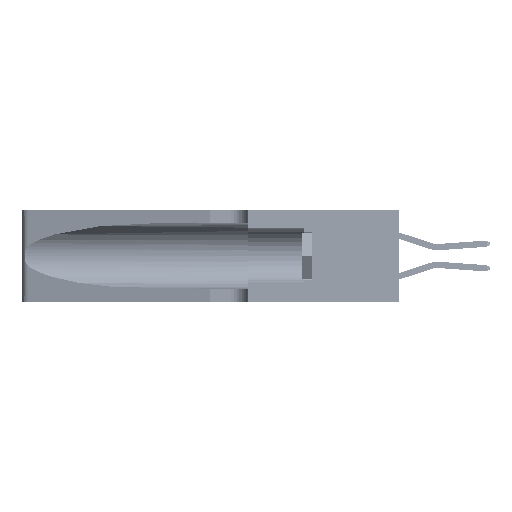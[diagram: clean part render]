
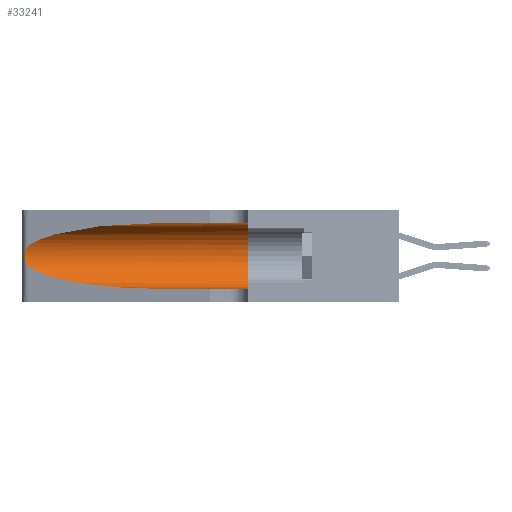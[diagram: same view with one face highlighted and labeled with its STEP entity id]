
A CAD part, left-side view. The second image highlights one B-rep face of the part: STEP entity #33241.
In plain terms, the highlighted cylindrical face has radius 3.308 mm (diameter 6.617 mm), a partial arc.
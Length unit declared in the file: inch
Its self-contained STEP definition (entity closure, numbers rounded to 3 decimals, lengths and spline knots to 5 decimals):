
#646 = CARTESIAN_POINT ( 'NONE',  ( 0.25555, 1.22994, 0.2215 ) ) ;
#1185 = DIRECTION ( 'NONE',  ( 0., -1., 0. ) ) ;
#1906 = VERTEX_POINT ( 'NONE', #7540 ) ;
#3377 = CIRCLE ( 'NONE', #4117, 0.13025 ) ;
#4117 = AXIS2_PLACEMENT_3D ( 'NONE', #32071, #7719, #36002 ) ;
#4422 = CARTESIAN_POINT ( 'NONE',  ( 0.25854, 1.2359, 0.20912 ) ) ;
#5748 = DIRECTION ( 'NONE',  ( 0., -1., 0. ) ) ;
#6317 = ORIENTED_EDGE ( 'NONE', *, *, #47443, .F. ) ;
#7099 = EDGE_CURVE ( 'NONE', #12326, #1906, #45762, .T. ) ;
#7443 = CARTESIAN_POINT ( 'NONE',  ( 0.18966, 0.96281, 0.05475 ) ) ;
#7540 = CARTESIAN_POINT ( 'NONE',  ( 0.1305, 0.35, 0.05475 ) ) ;
#7633 = CARTESIAN_POINT ( 'NONE',  ( 0.1305, 0.72297, 0.05475 ) ) ;
#7719 = DIRECTION ( 'NONE',  ( 0., 1., 0. ) ) ;
#8078 = CARTESIAN_POINT ( 'NONE',  ( 0.25487, 1.22718, 0.14631 ) ) ;
#8107 = EDGE_CURVE ( 'NONE', #32975, #12326, #27129, .T. ) ;
#8159 = ORIENTED_EDGE ( 'NONE', *, *, #41461, .F. ) ;
#8534 = CARTESIAN_POINT ( 'NONE',  ( 0.26075, 1.23896, 0.19203 ) ) ;
#9354 = AXIS2_PLACEMENT_3D ( 'NONE', #25885, #5748, #42400 ) ;
#9576 = FACE_OUTER_BOUND ( 'NONE', #43504, .T. ) ;
#12031 = CARTESIAN_POINT ( 'NONE',  ( 0.25487, 1.22718, 0.22369 ) ) ;
#12265 = CARTESIAN_POINT ( 'NONE',  ( 0.25639, 1.23184, 0.21858 ) ) ;
#12326 = VERTEX_POINT ( 'NONE', #42770 ) ;
#12560 = VERTEX_POINT ( 'NONE', #36156 ) ;
#16191 = CARTESIAN_POINT ( 'NONE',  ( 0.26017, 1.23833, 0.17102 ) ) ;
#16309 = CARTESIAN_POINT ( 'NONE',  ( 0.1305, 0.72297, 0.31525 ) ) ;
#16643 = DIRECTION ( 'NONE',  ( 0., -1., 0. ) ) ;
#18014 = EDGE_CURVE ( 'NONE', #12560, #32975, #37227, .T. ) ;
#18983 = CARTESIAN_POINT ( 'NONE',  ( 0.1305, 0.35, 0.31525 ) ) ;
#20297 = CARTESIAN_POINT ( 'NONE',  ( 0.25487, 1.22718, 0.14631 ) ) ;
#20485 = CARTESIAN_POINT ( 'NONE',  ( 0.25787, 1.23484, 0.2124 ) ) ;
#20595 = EDGE_CURVE ( 'NONE', #31140, #12560, #40496, .T. ) ;
#22894 = ORIENTED_EDGE ( 'NONE', *, *, #18014, .T. ) ;
#24033 = CARTESIAN_POINT ( 'NONE',  ( 0.2373, 1.15595, 0.08982 ) ) ;
#24583 = CARTESIAN_POINT ( 'NONE',  ( 0.25555, 1.22993, 0.14849 ) ) ;
#24810 = VECTOR ( 'NONE', #16643, 39.37008 ) ;
#25559 = CYLINDRICAL_SURFACE ( 'NONE', #9354, 0.13025 ) ;
#25770 = LINE ( 'NONE', #42508, #39709 ) ;
#25885 = CARTESIAN_POINT ( 'NONE',  ( 0.1305, 1.61858, 0.185 ) ) ;
#26699 = ORIENTED_EDGE ( 'NONE', *, *, #8107, .T. ) ;
#27129 =( BOUNDED_CURVE ( )  B_SPLINE_CURVE ( 3, ( #27952, #24033, #7443, #7633 ),
 .UNSPECIFIED., .F., .F. ) 
 B_SPLINE_CURVE_WITH_KNOTS ( ( 4, 4 ),
 ( 3.44316, 4.71239 ),
 .UNSPECIFIED. ) 
 CURVE ( )  GEOMETRIC_REPRESENTATION_ITEM ( )  RATIONAL_B_SPLINE_CURVE ( ( 1., 0.87, 0.87, 1. ) ) 
 REPRESENTATION_ITEM ( '' )  );
#27952 = CARTESIAN_POINT ( 'NONE',  ( 0.25487, 1.22718, 0.14631 ) ) ;
#29124 = CARTESIAN_POINT ( 'NONE',  ( 0.2373, 1.15595, 0.28018 ) ) ;
#31140 = VERTEX_POINT ( 'NONE', #41181 ) ;
#32071 = CARTESIAN_POINT ( 'NONE',  ( 0.1305, 0.35, 0.185 ) ) ;
#32891 = CARTESIAN_POINT ( 'NONE',  ( 0.26018, 1.23835, 0.19895 ) ) ;
#32975 = VERTEX_POINT ( 'NONE', #8078 ) ;
#33241 = ADVANCED_FACE ( 'NONE', ( #9576 ), #25559, .F. ) ;
#36002 = DIRECTION ( 'NONE',  ( 0., 0., 1. ) ) ;
#36156 = CARTESIAN_POINT ( 'NONE',  ( 0.25487, 1.22718, 0.22369 ) ) ;
#37008 = CARTESIAN_POINT ( 'NONE',  ( 0.26075, 1.23896, 0.178 ) ) ;
#37171 = CARTESIAN_POINT ( 'NONE',  ( 0.25639, 1.23186, 0.15144 ) ) ;
#37227 = B_SPLINE_CURVE_WITH_KNOTS ( 'NONE', 3,
 ( #44830, #646, #12265, #20485, #4422, #32891, #8534, #37008, #16191, #44662, #48946, #37171, #24583, #20297 ),
 .UNSPECIFIED., .F., .F.,
 ( 4, 2, 2, 2, 2, 2, 4 ),
 ( 0., 0.00027, 0.00053, 0.00107, 0.0016, 0.00187, 0.00214 ),
 .UNSPECIFIED. ) ;
#39709 = VECTOR ( 'NONE', #1185, 39.37008 ) ;
#40496 =( BOUNDED_CURVE ( )  B_SPLINE_CURVE ( 3, ( #16309, #40888, #29124, #12031 ),
 .UNSPECIFIED., .F., .T. ) 
 B_SPLINE_CURVE_WITH_KNOTS ( ( 4, 4 ),
 ( 1.5708, 2.84003 ),
 .UNSPECIFIED. ) 
 CURVE ( )  GEOMETRIC_REPRESENTATION_ITEM ( )  RATIONAL_B_SPLINE_CURVE ( ( 1., 0.87, 0.87, 1. ) ) 
 REPRESENTATION_ITEM ( '' )  );
#40888 = CARTESIAN_POINT ( 'NONE',  ( 0.18966, 0.96281, 0.31525 ) ) ;
#41038 = ORIENTED_EDGE ( 'NONE', *, *, #20595, .T. ) ;
#41181 = CARTESIAN_POINT ( 'NONE',  ( 0.1305, 0.72297, 0.31525 ) ) ;
#41461 = EDGE_CURVE ( 'NONE', #44089, #1906, #3377, .T. ) ;
#41737 = ORIENTED_EDGE ( 'NONE', *, *, #7099, .T. ) ;
#42400 = DIRECTION ( 'NONE',  ( 0., 0., -1. ) ) ;
#42508 = CARTESIAN_POINT ( 'NONE',  ( 0.1305, 1.61858, 0.31525 ) ) ;
#42770 = CARTESIAN_POINT ( 'NONE',  ( 0.1305, 0.72297, 0.05475 ) ) ;
#43504 = EDGE_LOOP ( 'NONE', ( #41038, #22894, #26699, #41737, #8159, #6317 ) ) ;
#44089 = VERTEX_POINT ( 'NONE', #18983 ) ;
#44662 = CARTESIAN_POINT ( 'NONE',  ( 0.25856, 1.23593, 0.16098 ) ) ;
#44830 = CARTESIAN_POINT ( 'NONE',  ( 0.25487, 1.22718, 0.22369 ) ) ;
#45762 = LINE ( 'NONE', #49929, #24810 ) ;
#47443 = EDGE_CURVE ( 'NONE', #31140, #44089, #25770, .T. ) ;
#48946 = CARTESIAN_POINT ( 'NONE',  ( 0.25789, 1.23486, 0.15765 ) ) ;
#49929 = CARTESIAN_POINT ( 'NONE',  ( 0.1305, 1.61858, 0.05475 ) ) ;
